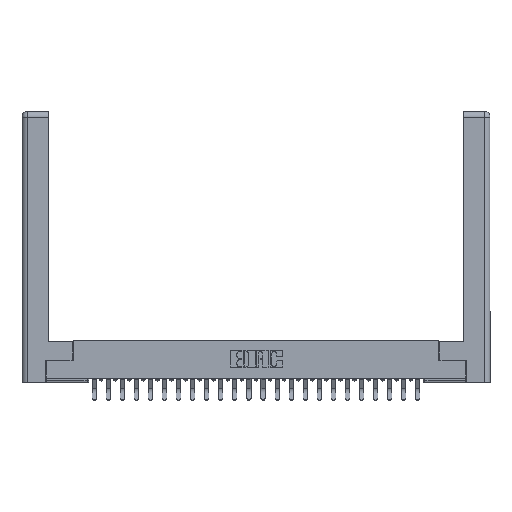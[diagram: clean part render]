
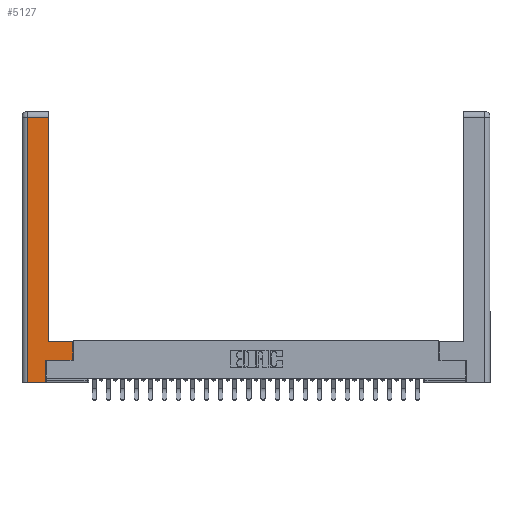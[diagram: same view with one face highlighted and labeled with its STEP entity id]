
A CAD part, top view. The second image highlights one B-rep face of the part: STEP entity #5127.
In plain terms, the highlighted planar face has unit normal (0, 0, 1).
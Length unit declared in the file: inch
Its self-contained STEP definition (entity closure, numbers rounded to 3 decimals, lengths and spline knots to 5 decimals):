
#54 = EDGE_CURVE ( 'NONE', #13617, #530, #21260, .T. ) ;
#141 = CARTESIAN_POINT ( 'NONE',  ( 0.295, 2.94, 0. ) ) ;
#435 = LINE ( 'NONE', #13303, #778 ) ;
#530 = VERTEX_POINT ( 'NONE', #9816 ) ;
#653 = CARTESIAN_POINT ( 'NONE',  ( 0.295, 0.45, 0. ) ) ;
#735 = FACE_OUTER_BOUND ( 'NONE', #23318, .T. ) ;
#778 = VECTOR ( 'NONE', #23501, 39.37008 ) ;
#865 = EDGE_CURVE ( 'NONE', #8855, #18713, #22471, .T. ) ;
#1144 = ORIENTED_EDGE ( 'NONE', *, *, #865, .T. ) ;
#2205 = CARTESIAN_POINT ( 'NONE',  ( 0.265, 0.245, 0. ) ) ;
#2211 = VERTEX_POINT ( 'NONE', #2205 ) ;
#2317 = ORIENTED_EDGE ( 'NONE', *, *, #12530, .T. ) ;
#2982 = CARTESIAN_POINT ( 'NONE',  ( 0.265, 0., 0. ) ) ;
#3168 = CARTESIAN_POINT ( 'NONE',  ( 0.565, 0.45, 0. ) ) ;
#3422 = VECTOR ( 'NONE', #18217, 39.37008 ) ;
#3830 = LINE ( 'NONE', #25300, #21301 ) ;
#5127 = ADVANCED_FACE ( 'NONE', ( #735 ), #19735, .F. ) ;
#5765 = ORIENTED_EDGE ( 'NONE', *, *, #18502, .T. ) ;
#6528 = LINE ( 'NONE', #2982, #19871 ) ;
#7409 = CARTESIAN_POINT ( 'NONE',  ( 0.565, 0.245, 0. ) ) ;
#8096 = CARTESIAN_POINT ( 'NONE',  ( 0.565, 0.245, 0. ) ) ;
#8724 = LINE ( 'NONE', #18088, #10354 ) ;
#8855 = VERTEX_POINT ( 'NONE', #7409 ) ;
#9816 = CARTESIAN_POINT ( 'NONE',  ( 0.0615, 2.94, 0. ) ) ;
#9963 = ORIENTED_EDGE ( 'NONE', *, *, #54, .T. ) ;
#10354 = VECTOR ( 'NONE', #18261, 39.37008 ) ;
#10694 = VECTOR ( 'NONE', #13181, 39.37008 ) ;
#11580 = CARTESIAN_POINT ( 'NONE',  ( 0., 0., 0. ) ) ;
#11967 = CARTESIAN_POINT ( 'NONE',  ( 0.0615, 0., 0. ) ) ;
#12034 = DIRECTION ( 'NONE',  ( 0., 0., -1. ) ) ;
#12530 = EDGE_CURVE ( 'NONE', #530, #18757, #8724, .T. ) ;
#12845 = CARTESIAN_POINT ( 'NONE',  ( 0.0615, 2.94, 0. ) ) ;
#13014 = CARTESIAN_POINT ( 'NONE',  ( 0.295, 3., 0. ) ) ;
#13181 = DIRECTION ( 'NONE',  ( 0., 1., 0. ) ) ;
#13303 = CARTESIAN_POINT ( 'NONE',  ( 0.265, 0.245, 0. ) ) ;
#13617 = VERTEX_POINT ( 'NONE', #141 ) ;
#14139 = CARTESIAN_POINT ( 'NONE',  ( 0.265, 0., 0. ) ) ;
#14721 = VERTEX_POINT ( 'NONE', #14139 ) ;
#15245 = VECTOR ( 'NONE', #25099, 39.37008 ) ;
#15538 = LINE ( 'NONE', #13014, #23162 ) ;
#15802 = LINE ( 'NONE', #8096, #3422 ) ;
#16333 = EDGE_CURVE ( 'NONE', #18713, #21529, #3830, .T. ) ;
#18088 = CARTESIAN_POINT ( 'NONE',  ( 0.0615, 0., 0. ) ) ;
#18217 = DIRECTION ( 'NONE',  ( 1., 0., 0. ) ) ;
#18261 = DIRECTION ( 'NONE',  ( 0., -1., 0. ) ) ;
#18502 = EDGE_CURVE ( 'NONE', #18757, #14721, #6528, .T. ) ;
#18713 = VERTEX_POINT ( 'NONE', #3168 ) ;
#18722 = EDGE_CURVE ( 'NONE', #14721, #2211, #435, .T. ) ;
#18757 = VERTEX_POINT ( 'NONE', #11967 ) ;
#18976 = ORIENTED_EDGE ( 'NONE', *, *, #16333, .T. ) ;
#19094 = DIRECTION ( 'NONE',  ( -1., 0., 0. ) ) ;
#19224 = ORIENTED_EDGE ( 'NONE', *, *, #24714, .T. ) ;
#19735 = PLANE ( 'NONE',  #22988 ) ;
#19871 = VECTOR ( 'NONE', #20826, 39.37008 ) ;
#20826 = DIRECTION ( 'NONE',  ( 1., 0., 0. ) ) ;
#21260 = LINE ( 'NONE', #12845, #15245 ) ;
#21301 = VECTOR ( 'NONE', #19094, 39.37008 ) ;
#21529 = VERTEX_POINT ( 'NONE', #653 ) ;
#22471 = LINE ( 'NONE', #25246, #10694 ) ;
#22988 = AXIS2_PLACEMENT_3D ( 'NONE', #11580, #12034, #26214 ) ;
#23162 = VECTOR ( 'NONE', #23213, 39.37008 ) ;
#23213 = DIRECTION ( 'NONE',  ( 0., 1., 0. ) ) ;
#23318 = EDGE_LOOP ( 'NONE', ( #19224, #9963, #2317, #5765, #25487, #23455, #1144, #18976 ) ) ;
#23455 = ORIENTED_EDGE ( 'NONE', *, *, #25621, .T. ) ;
#23501 = DIRECTION ( 'NONE',  ( 0., 1., 0. ) ) ;
#24714 = EDGE_CURVE ( 'NONE', #21529, #13617, #15538, .T. ) ;
#25099 = DIRECTION ( 'NONE',  ( -1., 0., 0. ) ) ;
#25246 = CARTESIAN_POINT ( 'NONE',  ( 0.565, 0.45, 0. ) ) ;
#25300 = CARTESIAN_POINT ( 'NONE',  ( 0.295, 0.45, 0. ) ) ;
#25487 = ORIENTED_EDGE ( 'NONE', *, *, #18722, .T. ) ;
#25621 = EDGE_CURVE ( 'NONE', #2211, #8855, #15802, .T. ) ;
#26214 = DIRECTION ( 'NONE',  ( -1., 0., 0. ) ) ;
